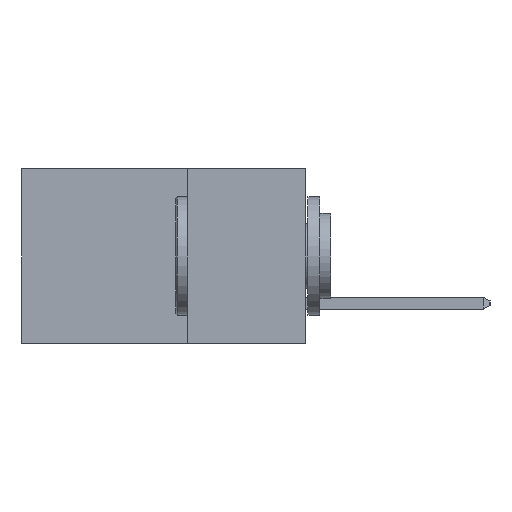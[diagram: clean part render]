
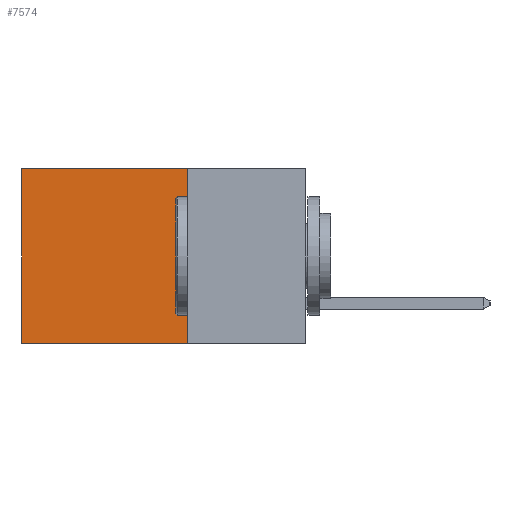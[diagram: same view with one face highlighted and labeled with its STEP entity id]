
A CAD part, left-side view. The second image highlights one B-rep face of the part: STEP entity #7574.
In plain terms, the highlighted planar face has unit normal (-1, 0, 0).
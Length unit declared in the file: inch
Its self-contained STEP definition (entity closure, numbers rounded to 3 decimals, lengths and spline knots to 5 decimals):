
#364 = ORIENTED_EDGE ( 'NONE', *, *, #9563, .F. ) ;
#1712 = AXIS2_PLACEMENT_3D ( 'NONE', #9519, #6449, #6282 ) ;
#2533 = CARTESIAN_POINT ( 'NONE',  ( 0.2615, 0.6, 0. ) ) ;
#2814 = LINE ( 'NONE', #20300, #7492 ) ;
#3261 = VERTEX_POINT ( 'NONE', #14210 ) ;
#3452 = ORIENTED_EDGE ( 'NONE', *, *, #6135, .T. ) ;
#4413 = EDGE_CURVE ( 'NONE', #4962, #8787, #22518, .T. ) ;
#4962 = VERTEX_POINT ( 'NONE', #18017 ) ;
#5537 = CARTESIAN_POINT ( 'NONE',  ( 0.2615, 0.25, -0.37 ) ) ;
#6135 = EDGE_CURVE ( 'NONE', #8787, #20476, #2814, .T. ) ;
#6282 = DIRECTION ( 'NONE',  ( 0., 0., -1. ) ) ;
#6343 = LINE ( 'NONE', #5537, #11619 ) ;
#6449 = DIRECTION ( 'NONE',  ( 1., 0., 0. ) ) ;
#6602 = PLANE ( 'NONE',  #1712 ) ;
#7222 = ORIENTED_EDGE ( 'NONE', *, *, #20716, .F. ) ;
#7252 = VECTOR ( 'NONE', #16641, 39.37008 ) ;
#7492 = VECTOR ( 'NONE', #20186, 39.37008 ) ;
#7574 = ADVANCED_FACE ( 'NONE', ( #24953 ), #6602, .F. ) ;
#7781 = ORIENTED_EDGE ( 'NONE', *, *, #4413, .T. ) ;
#8787 = VERTEX_POINT ( 'NONE', #2533 ) ;
#9519 = CARTESIAN_POINT ( 'NONE',  ( 0.2615, 0.25, -0.37 ) ) ;
#9563 = EDGE_CURVE ( 'NONE', #3261, #20476, #17140, .T. ) ;
#11619 = VECTOR ( 'NONE', #15384, 39.37008 ) ;
#13808 = CARTESIAN_POINT ( 'NONE',  ( 0.2615, 0.25, 0. ) ) ;
#14210 = CARTESIAN_POINT ( 'NONE',  ( 0.2615, 0.25, -0.37 ) ) ;
#14275 = DIRECTION ( 'NONE',  ( 0., 1., 0. ) ) ;
#15384 = DIRECTION ( 'NONE',  ( 0., 0., -1. ) ) ;
#16641 = DIRECTION ( 'NONE',  ( 0., 1., 0. ) ) ;
#16871 = VECTOR ( 'NONE', #14275, 39.37008 ) ;
#17102 = CARTESIAN_POINT ( 'NONE',  ( 0.2615, 0.25, -0.37 ) ) ;
#17140 = LINE ( 'NONE', #17102, #7252 ) ;
#17730 = EDGE_LOOP ( 'NONE', ( #3452, #364, #7222, #7781 ) ) ;
#18017 = CARTESIAN_POINT ( 'NONE',  ( 0.2615, 0.25, 0. ) ) ;
#20186 = DIRECTION ( 'NONE',  ( 0., 0., -1. ) ) ;
#20300 = CARTESIAN_POINT ( 'NONE',  ( 0.2615, 0.6, -0.37 ) ) ;
#20387 = CARTESIAN_POINT ( 'NONE',  ( 0.2615, 0.6, -0.37 ) ) ;
#20476 = VERTEX_POINT ( 'NONE', #20387 ) ;
#20716 = EDGE_CURVE ( 'NONE', #4962, #3261, #6343, .T. ) ;
#22518 = LINE ( 'NONE', #13808, #16871 ) ;
#24953 = FACE_OUTER_BOUND ( 'NONE', #17730, .T. ) ;
